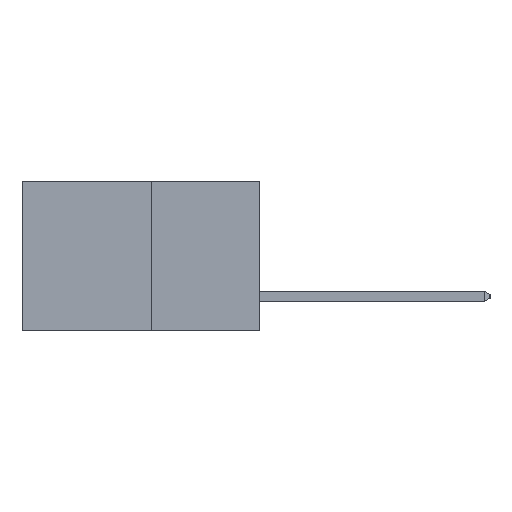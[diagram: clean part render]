
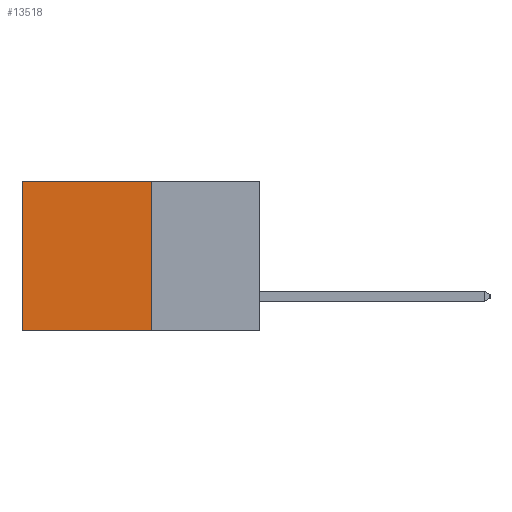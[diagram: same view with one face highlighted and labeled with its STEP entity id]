
A CAD part, left-side view. The second image highlights one B-rep face of the part: STEP entity #13518.
In plain terms, the highlighted planar face has unit normal (-1, 0, 0).
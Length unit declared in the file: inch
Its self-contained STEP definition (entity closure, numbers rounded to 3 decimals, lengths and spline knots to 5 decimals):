
#341 = CARTESIAN_POINT ( 'NONE',  ( 0.277, 0.59, -0.37 ) ) ;
#390 = DIRECTION ( 'NONE',  ( 0., 1., 0. ) ) ;
#1831 = DIRECTION ( 'NONE',  ( 0., 0., -1. ) ) ;
#2429 = CARTESIAN_POINT ( 'NONE',  ( 0.277, 0.59, -0.37 ) ) ;
#3415 = DIRECTION ( 'NONE',  ( 0., 1., 0. ) ) ;
#3577 = CARTESIAN_POINT ( 'NONE',  ( 0.277, 0.27, -0.37 ) ) ;
#3668 = VERTEX_POINT ( 'NONE', #14108 ) ;
#3720 = CARTESIAN_POINT ( 'NONE',  ( 0.277, 0.27, -0.37 ) ) ;
#4284 = VECTOR ( 'NONE', #4507, 39.37008 ) ;
#4507 = DIRECTION ( 'NONE',  ( 0., 0., -1. ) ) ;
#5160 = CARTESIAN_POINT ( 'NONE',  ( 0.277, 0.59, 0. ) ) ;
#5433 = VECTOR ( 'NONE', #3415, 39.37008 ) ;
#6116 = EDGE_CURVE ( 'NONE', #6814, #6179, #9271, .T. ) ;
#6179 = VERTEX_POINT ( 'NONE', #2429 ) ;
#6262 = FACE_OUTER_BOUND ( 'NONE', #8657, .T. ) ;
#6814 = VERTEX_POINT ( 'NONE', #3720 ) ;
#6928 = VECTOR ( 'NONE', #390, 39.37008 ) ;
#7585 = CARTESIAN_POINT ( 'NONE',  ( 0.277, 0.27, -0.37 ) ) ;
#8041 = ORIENTED_EDGE ( 'NONE', *, *, #6116, .F. ) ;
#8657 = EDGE_LOOP ( 'NONE', ( #11935, #8041, #15091, #15158 ) ) ;
#8669 = EDGE_CURVE ( 'NONE', #3668, #11031, #17999, .T. ) ;
#9031 = DIRECTION ( 'NONE',  ( 0., 0., -1. ) ) ;
#9120 = CARTESIAN_POINT ( 'NONE',  ( 0.277, 0.27, 0. ) ) ;
#9271 = LINE ( 'NONE', #3577, #5433 ) ;
#9515 = EDGE_CURVE ( 'NONE', #11031, #6179, #10858, .T. ) ;
#10427 = VECTOR ( 'NONE', #1831, 39.37008 ) ;
#10533 = LINE ( 'NONE', #14404, #4284 ) ;
#10858 = LINE ( 'NONE', #341, #10427 ) ;
#11031 = VERTEX_POINT ( 'NONE', #5160 ) ;
#11935 = ORIENTED_EDGE ( 'NONE', *, *, #9515, .T. ) ;
#13518 = ADVANCED_FACE ( 'NONE', ( #6262 ), #15949, .F. ) ;
#14108 = CARTESIAN_POINT ( 'NONE',  ( 0.277, 0.27, 0. ) ) ;
#14404 = CARTESIAN_POINT ( 'NONE',  ( 0.277, 0.27, -0.37 ) ) ;
#15091 = ORIENTED_EDGE ( 'NONE', *, *, #17122, .F. ) ;
#15158 = ORIENTED_EDGE ( 'NONE', *, *, #8669, .T. ) ;
#15949 = PLANE ( 'NONE',  #18087 ) ;
#17122 = EDGE_CURVE ( 'NONE', #3668, #6814, #10533, .T. ) ;
#17293 = DIRECTION ( 'NONE',  ( 1., 0., 0. ) ) ;
#17999 = LINE ( 'NONE', #9120, #6928 ) ;
#18087 = AXIS2_PLACEMENT_3D ( 'NONE', #7585, #17293, #9031 ) ;
